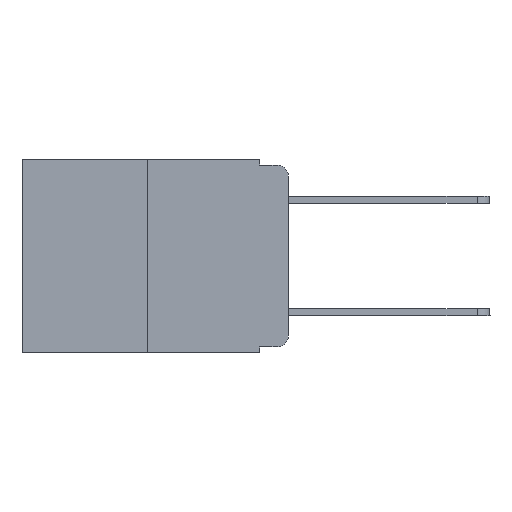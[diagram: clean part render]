
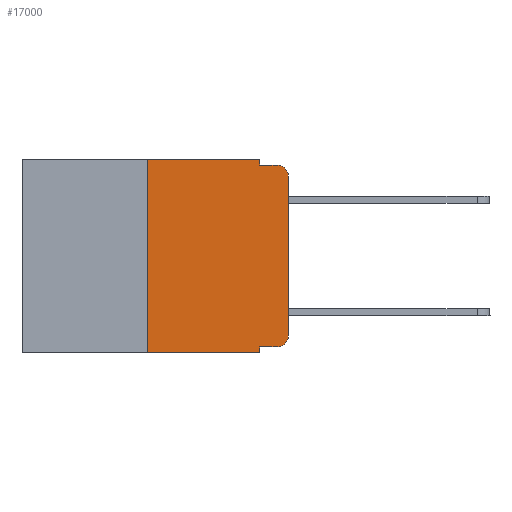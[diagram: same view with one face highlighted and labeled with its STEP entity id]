
A CAD part, left-side view. The second image highlights one B-rep face of the part: STEP entity #17000.
In plain terms, the highlighted planar face has unit normal (-1, 0, 0).
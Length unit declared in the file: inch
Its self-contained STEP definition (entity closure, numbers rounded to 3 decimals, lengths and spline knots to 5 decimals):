
#278 = EDGE_CURVE ( 'NONE', #16393, #17976, #24574, .T. ) ;
#748 = VERTEX_POINT ( 'NONE', #15140 ) ;
#808 = EDGE_LOOP ( 'NONE', ( #2343, #23199, #1694, #5650, #18436, #7087, #13713, #1073, #11419, #19960 ) ) ;
#880 = CARTESIAN_POINT ( 'NONE',  ( 0., 0.051, -0.343 ) ) ;
#1059 = DIRECTION ( 'NONE',  ( 1., 0., 0. ) ) ;
#1073 = ORIENTED_EDGE ( 'NONE', *, *, #278, .F. ) ;
#1277 = CARTESIAN_POINT ( 'NONE',  ( 0., 0.25, 0. ) ) ;
#1694 = ORIENTED_EDGE ( 'NONE', *, *, #9588, .F. ) ;
#2343 = ORIENTED_EDGE ( 'NONE', *, *, #15874, .T. ) ;
#2629 = CARTESIAN_POINT ( 'NONE',  ( 0., 0.473, 0. ) ) ;
#2862 = AXIS2_PLACEMENT_3D ( 'NONE', #12389, #23697, #20188 ) ;
#3435 = DIRECTION ( 'NONE',  ( 0., 0., 1. ) ) ;
#4220 = EDGE_CURVE ( 'NONE', #24328, #18942, #11550, .T. ) ;
#4841 = CIRCLE ( 'NONE', #2862, 0.02 ) ;
#5117 = CARTESIAN_POINT ( 'NONE',  ( 0., 0.02, -0.333 ) ) ;
#5650 = ORIENTED_EDGE ( 'NONE', *, *, #6651, .F. ) ;
#6651 = EDGE_CURVE ( 'NONE', #7581, #748, #13695, .T. ) ;
#6770 = VECTOR ( 'NONE', #3435, 39.37008 ) ;
#6996 = CARTESIAN_POINT ( 'NONE',  ( 0., 0.051, -0.333 ) ) ;
#7087 = ORIENTED_EDGE ( 'NONE', *, *, #4220, .F. ) ;
#7559 = EDGE_CURVE ( 'NONE', #24328, #17976, #11872, .T. ) ;
#7581 = VERTEX_POINT ( 'NONE', #14143 ) ;
#8397 = CARTESIAN_POINT ( 'NONE',  ( 0., 0.473, 0. ) ) ;
#8648 = DIRECTION ( 'NONE',  ( 0., 0., -1. ) ) ;
#9098 = VERTEX_POINT ( 'NONE', #5117 ) ;
#9588 = EDGE_CURVE ( 'NONE', #748, #19608, #20744, .T. ) ;
#9607 = CIRCLE ( 'NONE', #13626, 0.02 ) ;
#10531 = FACE_OUTER_BOUND ( 'NONE', #808, .T. ) ;
#10618 = EDGE_CURVE ( 'NONE', #18942, #7581, #19535, .T. ) ;
#11419 = ORIENTED_EDGE ( 'NONE', *, *, #14659, .T. ) ;
#11550 = LINE ( 'NONE', #18976, #21824 ) ;
#11816 = DIRECTION ( 'NONE',  ( 0., 0., -1. ) ) ;
#11848 = CARTESIAN_POINT ( 'NONE',  ( 0., 0.02, -0.01 ) ) ;
#11872 = LINE ( 'NONE', #19538, #14150 ) ;
#12389 = CARTESIAN_POINT ( 'NONE',  ( 0., 0.02, -0.313 ) ) ;
#12417 = PLANE ( 'NONE',  #18449 ) ;
#12693 = CARTESIAN_POINT ( 'NONE',  ( 0., 0., 0. ) ) ;
#12835 = CARTESIAN_POINT ( 'NONE',  ( 0., 0., -0.03 ) ) ;
#13398 = DIRECTION ( 'NONE',  ( 0., 0., -1. ) ) ;
#13626 = AXIS2_PLACEMENT_3D ( 'NONE', #17842, #23848, #8648 ) ;
#13695 = LINE ( 'NONE', #21370, #18098 ) ;
#13713 = ORIENTED_EDGE ( 'NONE', *, *, #7559, .T. ) ;
#14143 = CARTESIAN_POINT ( 'NONE',  ( 0., 0.051, 0. ) ) ;
#14150 = VECTOR ( 'NONE', #19795, 39.37008 ) ;
#14193 = VERTEX_POINT ( 'NONE', #12835 ) ;
#14401 = CARTESIAN_POINT ( 'NONE',  ( 0., 0., -0.313 ) ) ;
#14659 = EDGE_CURVE ( 'NONE', #16393, #9098, #17099, .T. ) ;
#15010 = VECTOR ( 'NONE', #20664, 39.37008 ) ;
#15140 = CARTESIAN_POINT ( 'NONE',  ( 0., 0.051, -0.01 ) ) ;
#15450 = CARTESIAN_POINT ( 'NONE',  ( 0., 0.051, -0.333 ) ) ;
#15533 = DIRECTION ( 'NONE',  ( 0., -1., 0. ) ) ;
#15874 = EDGE_CURVE ( 'NONE', #23465, #14193, #22115, .T. ) ;
#16393 = VERTEX_POINT ( 'NONE', #6996 ) ;
#16990 = CARTESIAN_POINT ( 'NONE',  ( 0., 0.051, -0.01 ) ) ;
#17000 = ADVANCED_FACE ( 'NONE', ( #10531 ), #12417, .F. ) ;
#17018 = EDGE_CURVE ( 'NONE', #14193, #19608, #9607, .T. ) ;
#17099 = LINE ( 'NONE', #15450, #21567 ) ;
#17114 = DIRECTION ( 'NONE',  ( 0., 0., 1. ) ) ;
#17340 = DIRECTION ( 'NONE',  ( 0., -1., 0. ) ) ;
#17842 = CARTESIAN_POINT ( 'NONE',  ( 0., 0.02, -0.03 ) ) ;
#17953 = DIRECTION ( 'NONE',  ( 0., 0., -1. ) ) ;
#17976 = VERTEX_POINT ( 'NONE', #880 ) ;
#18098 = VECTOR ( 'NONE', #11816, 39.37008 ) ;
#18192 = CARTESIAN_POINT ( 'NONE',  ( 0., 0.25, -0.343 ) ) ;
#18436 = ORIENTED_EDGE ( 'NONE', *, *, #10618, .F. ) ;
#18449 = AXIS2_PLACEMENT_3D ( 'NONE', #8397, #1059, #17953 ) ;
#18822 = EDGE_CURVE ( 'NONE', #9098, #23465, #4841, .T. ) ;
#18942 = VERTEX_POINT ( 'NONE', #1277 ) ;
#18976 = CARTESIAN_POINT ( 'NONE',  ( 0., 0.25, 0. ) ) ;
#19535 = LINE ( 'NONE', #2629, #20667 ) ;
#19538 = CARTESIAN_POINT ( 'NONE',  ( 0., 0.473, -0.343 ) ) ;
#19608 = VERTEX_POINT ( 'NONE', #11848 ) ;
#19795 = DIRECTION ( 'NONE',  ( 0., -1., 0. ) ) ;
#19960 = ORIENTED_EDGE ( 'NONE', *, *, #18822, .T. ) ;
#20188 = DIRECTION ( 'NONE',  ( 0., 0., -1. ) ) ;
#20664 = DIRECTION ( 'NONE',  ( 0., -1., 0. ) ) ;
#20667 = VECTOR ( 'NONE', #15533, 39.37008 ) ;
#20744 = LINE ( 'NONE', #16990, #15010 ) ;
#20814 = CARTESIAN_POINT ( 'NONE',  ( 0., 0.051, 0. ) ) ;
#21357 = VECTOR ( 'NONE', #13398, 39.37008 ) ;
#21370 = CARTESIAN_POINT ( 'NONE',  ( 0., 0.051, 0. ) ) ;
#21567 = VECTOR ( 'NONE', #17340, 39.37008 ) ;
#21824 = VECTOR ( 'NONE', #17114, 39.37008 ) ;
#22115 = LINE ( 'NONE', #12693, #6770 ) ;
#23199 = ORIENTED_EDGE ( 'NONE', *, *, #17018, .T. ) ;
#23465 = VERTEX_POINT ( 'NONE', #14401 ) ;
#23697 = DIRECTION ( 'NONE',  ( -1., 0., 0. ) ) ;
#23848 = DIRECTION ( 'NONE',  ( -1., 0., 0. ) ) ;
#24328 = VERTEX_POINT ( 'NONE', #18192 ) ;
#24574 = LINE ( 'NONE', #20814, #21357 ) ;
